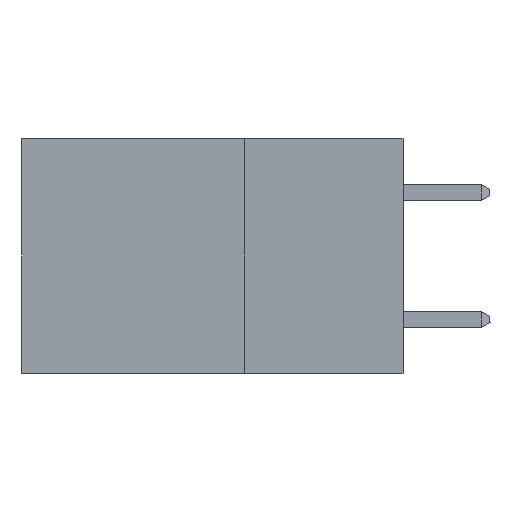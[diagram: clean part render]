
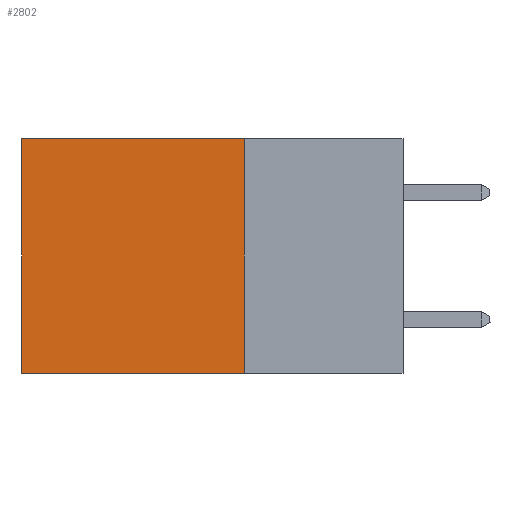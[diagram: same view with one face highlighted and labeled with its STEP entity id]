
A CAD part, left-side view. The second image highlights one B-rep face of the part: STEP entity #2802.
In plain terms, the highlighted planar face has unit normal (-1, 0, 0).
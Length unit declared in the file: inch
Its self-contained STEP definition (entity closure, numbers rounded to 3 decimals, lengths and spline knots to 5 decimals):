
#709 = EDGE_CURVE ( 'NONE', #12720, #3336, #16556, .T. ) ;
#829 = CARTESIAN_POINT ( 'NONE',  ( 0.2875, 0.25, 0. ) ) ;
#1802 = EDGE_CURVE ( 'NONE', #14046, #12720, #15691, .T. ) ;
#2397 = EDGE_LOOP ( 'NONE', ( #4886, #9824, #12919, #15824 ) ) ;
#2802 = ADVANCED_FACE ( 'NONE', ( #7369 ), #5824, .F. ) ;
#3316 = LINE ( 'NONE', #3870, #6333 ) ;
#3336 = VERTEX_POINT ( 'NONE', #4465 ) ;
#3536 = DIRECTION ( 'NONE',  ( 1., 0., 0. ) ) ;
#3870 = CARTESIAN_POINT ( 'NONE',  ( 0.2875, 0.25, -0.37 ) ) ;
#3949 = CARTESIAN_POINT ( 'NONE',  ( 0.2875, 0.6, 0. ) ) ;
#4343 = DIRECTION ( 'NONE',  ( 0., 0., -1. ) ) ;
#4465 = CARTESIAN_POINT ( 'NONE',  ( 0.2875, 0.6, -0.37 ) ) ;
#4886 = ORIENTED_EDGE ( 'NONE', *, *, #709, .T. ) ;
#5513 = CARTESIAN_POINT ( 'NONE',  ( 0.2875, 0.25, -0.37 ) ) ;
#5824 = PLANE ( 'NONE',  #11159 ) ;
#6333 = VECTOR ( 'NONE', #11540, 39.37008 ) ;
#7246 = CARTESIAN_POINT ( 'NONE',  ( 0.2875, 0.25, 0. ) ) ;
#7369 = FACE_OUTER_BOUND ( 'NONE', #2397, .T. ) ;
#7829 = CARTESIAN_POINT ( 'NONE',  ( 0.2875, 0.25, 0. ) ) ;
#9403 = DIRECTION ( 'NONE',  ( 0., 1., 0. ) ) ;
#9423 = EDGE_CURVE ( 'NONE', #16318, #3336, #3316, .T. ) ;
#9824 = ORIENTED_EDGE ( 'NONE', *, *, #9423, .F. ) ;
#9944 = DIRECTION ( 'NONE',  ( 0., 0., -1. ) ) ;
#10833 = VECTOR ( 'NONE', #4343, 39.37008 ) ;
#10902 = CARTESIAN_POINT ( 'NONE',  ( 0.2875, 0.25, 0. ) ) ;
#11031 = VECTOR ( 'NONE', #9403, 39.37008 ) ;
#11070 = VECTOR ( 'NONE', #11851, 39.37008 ) ;
#11159 = AXIS2_PLACEMENT_3D ( 'NONE', #7246, #3536, #9944 ) ;
#11540 = DIRECTION ( 'NONE',  ( 0., 1., 0. ) ) ;
#11851 = DIRECTION ( 'NONE',  ( 0., 0., -1. ) ) ;
#12720 = VERTEX_POINT ( 'NONE', #14846 ) ;
#12919 = ORIENTED_EDGE ( 'NONE', *, *, #15940, .F. ) ;
#14046 = VERTEX_POINT ( 'NONE', #829 ) ;
#14846 = CARTESIAN_POINT ( 'NONE',  ( 0.2875, 0.6, 0. ) ) ;
#15516 = LINE ( 'NONE', #10902, #10833 ) ;
#15691 = LINE ( 'NONE', #7829, #11031 ) ;
#15824 = ORIENTED_EDGE ( 'NONE', *, *, #1802, .T. ) ;
#15940 = EDGE_CURVE ( 'NONE', #14046, #16318, #15516, .T. ) ;
#16318 = VERTEX_POINT ( 'NONE', #5513 ) ;
#16556 = LINE ( 'NONE', #3949, #11070 ) ;
